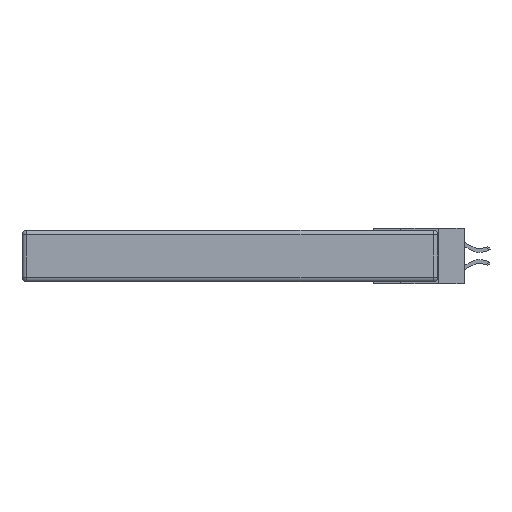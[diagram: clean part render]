
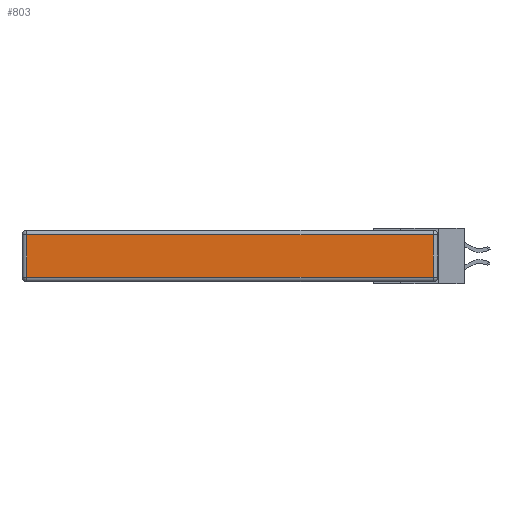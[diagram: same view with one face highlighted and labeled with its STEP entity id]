
A CAD part, left-side view. The second image highlights one B-rep face of the part: STEP entity #803.
In plain terms, the highlighted planar face has unit normal (-1, 0, 0).
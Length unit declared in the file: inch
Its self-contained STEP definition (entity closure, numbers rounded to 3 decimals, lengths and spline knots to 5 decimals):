
#5 = EDGE_LOOP ( 'NONE', ( #22380, #15986, #21254, #20 ) ) ;
#20 = ORIENTED_EDGE ( 'NONE', *, *, #9501, .T. ) ;
#803 = ADVANCED_FACE ( 'NONE', ( #6258 ), #9438, .T. ) ;
#863 = VECTOR ( 'NONE', #17988, 39.37008 ) ;
#1389 = EDGE_CURVE ( 'NONE', #6758, #22235, #2647, .T. ) ;
#1443 = DIRECTION ( 'NONE',  ( 0., 0., 1. ) ) ;
#2647 = LINE ( 'NONE', #6171, #7199 ) ;
#2737 = LINE ( 'NONE', #24339, #19762 ) ;
#3141 = VECTOR ( 'NONE', #13319, 39.37008 ) ;
#3177 = VERTEX_POINT ( 'NONE', #7597 ) ;
#3546 = CARTESIAN_POINT ( 'NONE',  ( 0., 2.75, -0.03 ) ) ;
#5070 = VERTEX_POINT ( 'NONE', #10499 ) ;
#6171 = CARTESIAN_POINT ( 'NONE',  ( 0., 0.03, -0.343 ) ) ;
#6258 = FACE_OUTER_BOUND ( 'NONE', #5, .T. ) ;
#6758 = VERTEX_POINT ( 'NONE', #22480 ) ;
#7199 = VECTOR ( 'NONE', #12081, 39.37008 ) ;
#7597 = CARTESIAN_POINT ( 'NONE',  ( 0., 2.72, -0.03 ) ) ;
#9438 = PLANE ( 'NONE',  #17152 ) ;
#9501 = EDGE_CURVE ( 'NONE', #3177, #5070, #2737, .T. ) ;
#9609 = DIRECTION ( 'NONE',  ( -1., 0., 0. ) ) ;
#10391 = CARTESIAN_POINT ( 'NONE',  ( 0., 0., -0.313 ) ) ;
#10499 = CARTESIAN_POINT ( 'NONE',  ( 0., 2.72, -0.313 ) ) ;
#11751 = CARTESIAN_POINT ( 'NONE',  ( 0., 0.03, -0.03 ) ) ;
#12081 = DIRECTION ( 'NONE',  ( 0., 0., 1. ) ) ;
#13319 = DIRECTION ( 'NONE',  ( 0., -1., 0. ) ) ;
#14707 = LINE ( 'NONE', #10391, #3141 ) ;
#15986 = ORIENTED_EDGE ( 'NONE', *, *, #1389, .T. ) ;
#17152 = AXIS2_PLACEMENT_3D ( 'NONE', #21926, #9609, #1443 ) ;
#17988 = DIRECTION ( 'NONE',  ( 0., 1., 0. ) ) ;
#18501 = EDGE_CURVE ( 'NONE', #22235, #3177, #20476, .T. ) ;
#19762 = VECTOR ( 'NONE', #22345, 39.37008 ) ;
#20476 = LINE ( 'NONE', #3546, #863 ) ;
#21254 = ORIENTED_EDGE ( 'NONE', *, *, #18501, .T. ) ;
#21926 = CARTESIAN_POINT ( 'NONE',  ( 0., 0., -0.343 ) ) ;
#22235 = VERTEX_POINT ( 'NONE', #11751 ) ;
#22345 = DIRECTION ( 'NONE',  ( 0., 0., -1. ) ) ;
#22380 = ORIENTED_EDGE ( 'NONE', *, *, #22896, .T. ) ;
#22480 = CARTESIAN_POINT ( 'NONE',  ( 0., 0.03, -0.313 ) ) ;
#22896 = EDGE_CURVE ( 'NONE', #5070, #6758, #14707, .T. ) ;
#24339 = CARTESIAN_POINT ( 'NONE',  ( 0., 2.72, -0.343 ) ) ;
